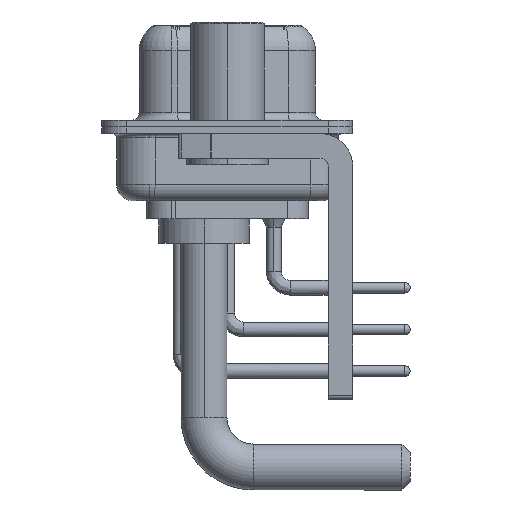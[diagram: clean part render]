
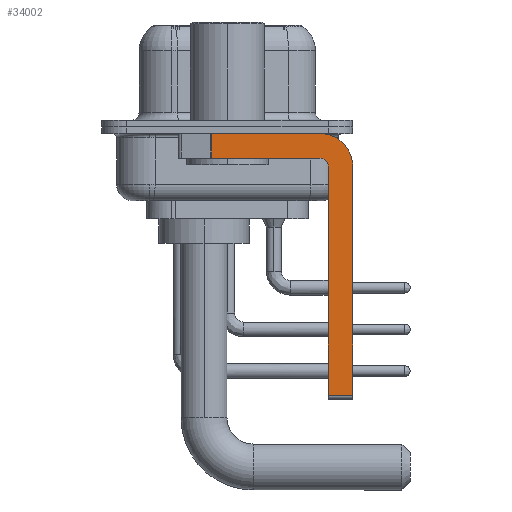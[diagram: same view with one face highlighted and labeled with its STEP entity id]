
A CAD part, left-side view. The second image highlights one B-rep face of the part: STEP entity #34002.
In plain terms, the highlighted planar face has unit normal (-1, 0, 0).
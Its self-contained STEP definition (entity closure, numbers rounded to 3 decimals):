
#320 = PLANE ( 'NONE',  #26640 ) ;
#388 = EDGE_CURVE ( 'NONE', #12323, #23567, #14314, .T. ) ;
#402 = CARTESIAN_POINT ( 'NONE',  ( -2.9, 0.978, -0.4 ) ) ;
#1319 = CARTESIAN_POINT ( 'NONE',  ( -2.9, -5.65, -0.4 ) ) ;
#2369 = CARTESIAN_POINT ( 'NONE',  ( -2.9, -5.65, -1.9 ) ) ;
#2382 = DIRECTION ( 'NONE',  ( 0., 0., -1. ) ) ;
#2654 = DIRECTION ( 'NONE',  ( 0., 0., 1. ) ) ;
#4535 = VERTEX_POINT ( 'NONE', #2369 ) ;
#6035 = CIRCLE ( 'NONE', #19020, 0.5 ) ;
#6331 = DIRECTION ( 'NONE',  ( 0., 0., -1. ) ) ;
#7148 = DIRECTION ( 'NONE',  ( 0., 1., 0. ) ) ;
#7428 = ORIENTED_EDGE ( 'NONE', *, *, #9970, .F. ) ;
#7917 = CIRCLE ( 'NONE', #27376, 2. ) ;
#8592 = ORIENTED_EDGE ( 'NONE', *, *, #388, .T. ) ;
#9958 = LINE ( 'NONE', #24911, #17753 ) ;
#9970 = EDGE_CURVE ( 'NONE', #20747, #23567, #10270, .T. ) ;
#10270 = LINE ( 'NONE', #18597, #22283 ) ;
#11368 = DIRECTION ( 'NONE',  ( 0., -1., 0. ) ) ;
#11600 = DIRECTION ( 'NONE',  ( 1., 0., 0. ) ) ;
#12313 = VERTEX_POINT ( 'NONE', #1319 ) ;
#12323 = VERTEX_POINT ( 'NONE', #35077 ) ;
#12840 = DIRECTION ( 'NONE',  ( 0., -1., 0. ) ) ;
#13124 = VERTEX_POINT ( 'NONE', #402 ) ;
#13565 = LINE ( 'NONE', #21351, #22082 ) ;
#13696 = ORIENTED_EDGE ( 'NONE', *, *, #26575, .F. ) ;
#14314 = LINE ( 'NONE', #25376, #17853 ) ;
#14728 = FACE_OUTER_BOUND ( 'NONE', #22582, .T. ) ;
#15331 = EDGE_CURVE ( 'NONE', #13124, #24343, #9958, .T. ) ;
#15372 = ORIENTED_EDGE ( 'NONE', *, *, #36258, .F. ) ;
#15530 = VERTEX_POINT ( 'NONE', #25645 ) ;
#15660 = LINE ( 'NONE', #18630, #29783 ) ;
#16463 = EDGE_CURVE ( 'NONE', #15530, #4535, #6035, .T. ) ;
#17342 = CARTESIAN_POINT ( 'NONE',  ( -2.9, -5.65, -2.4 ) ) ;
#17753 = VECTOR ( 'NONE', #2382, 1000. ) ;
#17853 = VECTOR ( 'NONE', #11368, 1000. ) ;
#17941 = VECTOR ( 'NONE', #2654, 1000. ) ;
#18451 = DIRECTION ( 'NONE',  ( -1., 0., 0. ) ) ;
#18597 = CARTESIAN_POINT ( 'NONE',  ( -2.9, -7.65, -2.4 ) ) ;
#18630 = CARTESIAN_POINT ( 'NONE',  ( -2.9, -5.65, -1.9 ) ) ;
#19020 = AXIS2_PLACEMENT_3D ( 'NONE', #32415, #18451, #24509 ) ;
#20205 = CARTESIAN_POINT ( 'NONE',  ( -2.9, -6.15, -16.6 ) ) ;
#20747 = VERTEX_POINT ( 'NONE', #21772 ) ;
#21351 = CARTESIAN_POINT ( 'NONE',  ( -2.9, 3., -0.4 ) ) ;
#21545 = DIRECTION ( 'NONE',  ( 0., 0., -1. ) ) ;
#21772 = CARTESIAN_POINT ( 'NONE',  ( -2.9, -7.65, -2.4 ) ) ;
#22082 = VECTOR ( 'NONE', #12840, 1000. ) ;
#22283 = VECTOR ( 'NONE', #21545, 1000. ) ;
#22582 = EDGE_LOOP ( 'NONE', ( #13696, #25127, #33998, #25324, #30838, #8592, #7428, #15372 ) ) ;
#23498 = DIRECTION ( 'NONE',  ( 1., 0., 0. ) ) ;
#23567 = VERTEX_POINT ( 'NONE', #31879 ) ;
#24343 = VERTEX_POINT ( 'NONE', #27856 ) ;
#24509 = DIRECTION ( 'NONE',  ( 0., 0., 1. ) ) ;
#24911 = CARTESIAN_POINT ( 'NONE',  ( -2.9, 0.978, -1.9 ) ) ;
#25127 = ORIENTED_EDGE ( 'NONE', *, *, #15331, .T. ) ;
#25324 = ORIENTED_EDGE ( 'NONE', *, *, #16463, .F. ) ;
#25376 = CARTESIAN_POINT ( 'NONE',  ( -2.9, -5.65, -16.35 ) ) ;
#25645 = CARTESIAN_POINT ( 'NONE',  ( -2.9, -6.15, -2.4 ) ) ;
#26575 = EDGE_CURVE ( 'NONE', #13124, #12313, #13565, .T. ) ;
#26640 = AXIS2_PLACEMENT_3D ( 'NONE', #17342, #11600, #28210 ) ;
#27247 = EDGE_CURVE ( 'NONE', #4535, #24343, #15660, .T. ) ;
#27376 = AXIS2_PLACEMENT_3D ( 'NONE', #29029, #23498, #6331 ) ;
#27856 = CARTESIAN_POINT ( 'NONE',  ( -2.9, 0.978, -1.9 ) ) ;
#28210 = DIRECTION ( 'NONE',  ( 0., 0., -1. ) ) ;
#29029 = CARTESIAN_POINT ( 'NONE',  ( -2.9, -5.65, -2.4 ) ) ;
#29783 = VECTOR ( 'NONE', #7148, 1000. ) ;
#30838 = ORIENTED_EDGE ( 'NONE', *, *, #35802, .F. ) ;
#31879 = CARTESIAN_POINT ( 'NONE',  ( -2.9, -7.65, -16.35 ) ) ;
#32415 = CARTESIAN_POINT ( 'NONE',  ( -2.9, -5.65, -2.4 ) ) ;
#33998 = ORIENTED_EDGE ( 'NONE', *, *, #27247, .F. ) ;
#34002 = ADVANCED_FACE ( 'NONE', ( #14728 ), #320, .F. ) ;
#34178 = LINE ( 'NONE', #20205, #17941 ) ;
#35077 = CARTESIAN_POINT ( 'NONE',  ( -2.9, -6.15, -16.35 ) ) ;
#35802 = EDGE_CURVE ( 'NONE', #12323, #15530, #34178, .T. ) ;
#36258 = EDGE_CURVE ( 'NONE', #12313, #20747, #7917, .T. ) ;
